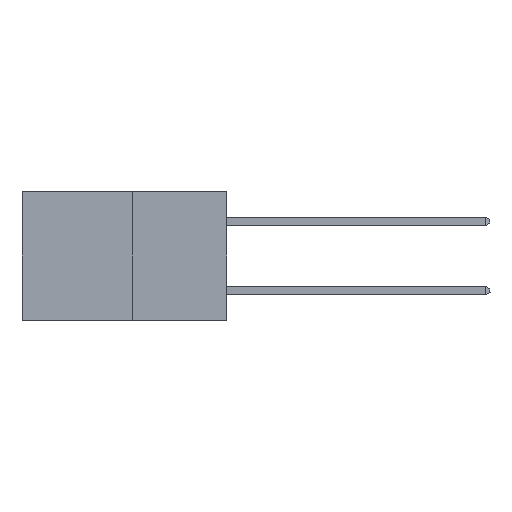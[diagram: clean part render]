
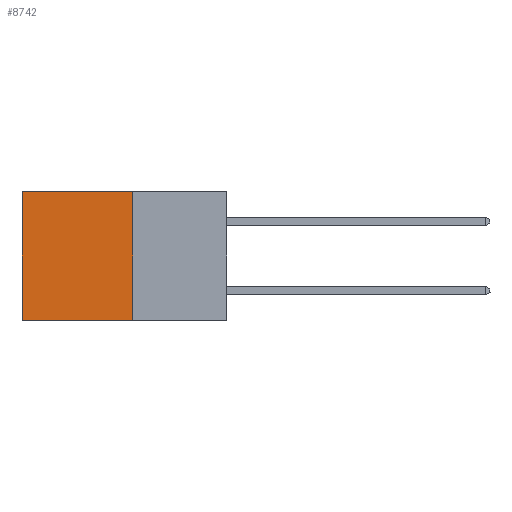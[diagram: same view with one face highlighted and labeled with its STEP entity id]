
A CAD part, left-side view. The second image highlights one B-rep face of the part: STEP entity #8742.
In plain terms, the highlighted planar face has unit normal (-1, 0, 0).
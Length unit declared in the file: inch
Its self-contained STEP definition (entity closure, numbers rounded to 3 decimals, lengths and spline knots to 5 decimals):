
#1029 = CARTESIAN_POINT ( 'NONE',  ( 0.277, 0.27, -0.37 ) ) ;
#1054 = ORIENTED_EDGE ( 'NONE', *, *, #2484, .F. ) ;
#1671 = CARTESIAN_POINT ( 'NONE',  ( 0.277, 0.59, 0. ) ) ;
#2450 = EDGE_CURVE ( 'NONE', #2988, #4259, #5111, .T. ) ;
#2484 = EDGE_CURVE ( 'NONE', #4259, #8731, #2576, .T. ) ;
#2490 = LINE ( 'NONE', #3477, #6271 ) ;
#2576 = LINE ( 'NONE', #1029, #6362 ) ;
#2647 = ORIENTED_EDGE ( 'NONE', *, *, #5398, .T. ) ;
#2988 = VERTEX_POINT ( 'NONE', #6799 ) ;
#3139 = EDGE_LOOP ( 'NONE', ( #2647, #1054, #3655, #7575 ) ) ;
#3398 = DIRECTION ( 'NONE',  ( 0., 1., 0. ) ) ;
#3477 = CARTESIAN_POINT ( 'NONE',  ( 0.277, 0.27, 0. ) ) ;
#3655 = ORIENTED_EDGE ( 'NONE', *, *, #2450, .F. ) ;
#3956 = FACE_OUTER_BOUND ( 'NONE', #3139, .T. ) ;
#4259 = VERTEX_POINT ( 'NONE', #7170 ) ;
#4932 = VECTOR ( 'NONE', #7895, 39.37008 ) ;
#5111 = LINE ( 'NONE', #7250, #6826 ) ;
#5296 = DIRECTION ( 'NONE',  ( 0., 0., -1. ) ) ;
#5303 = DIRECTION ( 'NONE',  ( 1., 0., 0. ) ) ;
#5329 = CARTESIAN_POINT ( 'NONE',  ( 0.277, 0.27, -0.37 ) ) ;
#5339 = PLANE ( 'NONE',  #6745 ) ;
#5373 = CARTESIAN_POINT ( 'NONE',  ( 0.277, 0.59, -0.37 ) ) ;
#5398 = EDGE_CURVE ( 'NONE', #9636, #8731, #6662, .T. ) ;
#6271 = VECTOR ( 'NONE', #3398, 39.37008 ) ;
#6362 = VECTOR ( 'NONE', #8304, 39.37008 ) ;
#6659 = CARTESIAN_POINT ( 'NONE',  ( 0.277, 0.59, -0.37 ) ) ;
#6662 = LINE ( 'NONE', #6659, #4932 ) ;
#6745 = AXIS2_PLACEMENT_3D ( 'NONE', #5329, #5303, #5296 ) ;
#6799 = CARTESIAN_POINT ( 'NONE',  ( 0.277, 0.27, 0. ) ) ;
#6826 = VECTOR ( 'NONE', #9789, 39.37008 ) ;
#7097 = EDGE_CURVE ( 'NONE', #2988, #9636, #2490, .T. ) ;
#7170 = CARTESIAN_POINT ( 'NONE',  ( 0.277, 0.27, -0.37 ) ) ;
#7250 = CARTESIAN_POINT ( 'NONE',  ( 0.277, 0.27, -0.37 ) ) ;
#7575 = ORIENTED_EDGE ( 'NONE', *, *, #7097, .T. ) ;
#7895 = DIRECTION ( 'NONE',  ( 0., 0., -1. ) ) ;
#8304 = DIRECTION ( 'NONE',  ( 0., 1., 0. ) ) ;
#8731 = VERTEX_POINT ( 'NONE', #5373 ) ;
#8742 = ADVANCED_FACE ( 'NONE', ( #3956 ), #5339, .F. ) ;
#9636 = VERTEX_POINT ( 'NONE', #1671 ) ;
#9789 = DIRECTION ( 'NONE',  ( 0., 0., -1. ) ) ;
